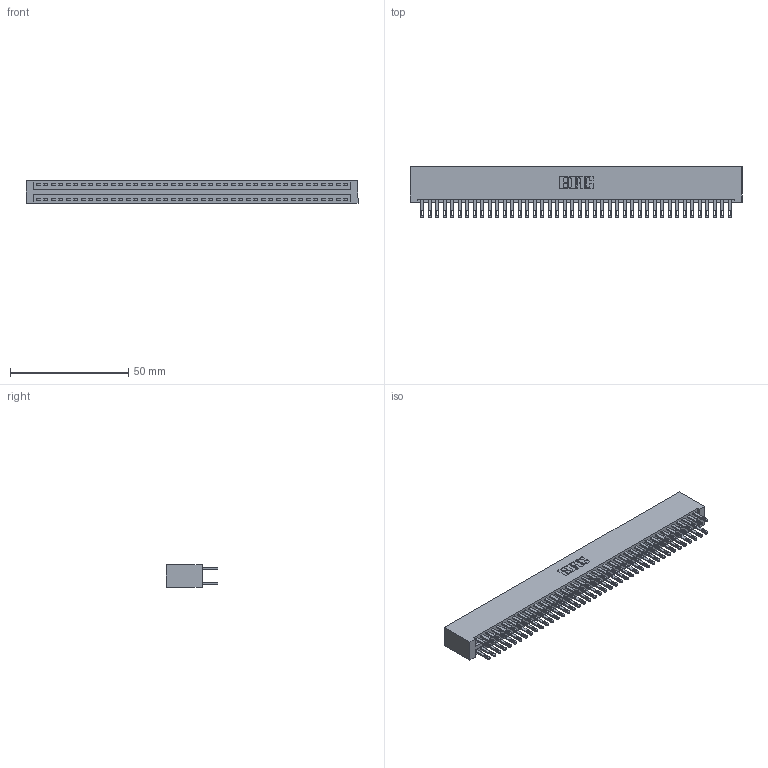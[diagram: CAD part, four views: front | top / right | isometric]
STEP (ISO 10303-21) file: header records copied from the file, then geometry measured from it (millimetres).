
FILE_DESCRIPTION (( 'STEP AP203' ), '1' );
FILE_NAME ('346-084-500-201.STEP', '2018-08-29T10:34:57', ( '' ), ( '' ), 'SwSTEP 2.0', 'SolidWorks 2016', '' );
FILE_SCHEMA (( 'CONFIG_CONTROL_DESIGN' ));
Length unit declared in the file: inch
Products named in the file (3): 346 Part_No Mounting Lugs; 345-292-001_345-293-100; 346-084-500-201
Assembly tree (85 placements, depth 2):
  346-084-500-201
    346 Part_No Mounting Lugs
    345-292-001_345-293-100  x84
Bounding box: 140.59 x 21.84 x 9.4 mm (x, y, z)
Volume: 14539.1 mm3; surface area: 21027.4 mm2
Topology: 85 solids, 85 shells, 4146 faces, 12653 edges, 8434 vertices
Faces by surface type: plane 2508, cylinder 1638
Entity records: 27063 total; most frequent: CARTESIAN_POINT 4456, ORIENTED_EDGE 4390, DIRECTION 3975, EDGE_CURVE 2195, LINE 1899, VECTOR 1899, VERTEX_POINT 1462, AXIS2_PLACEMENT_3D 1038
